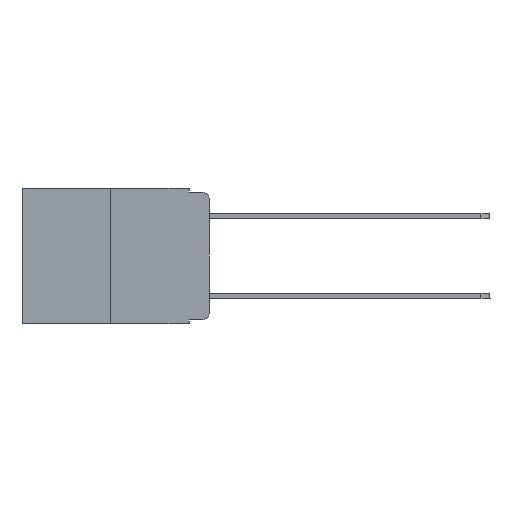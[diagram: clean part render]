
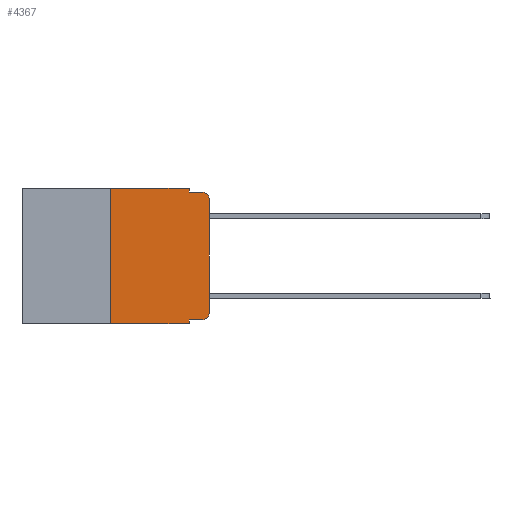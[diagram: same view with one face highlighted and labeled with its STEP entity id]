
A CAD part, left-side view. The second image highlights one B-rep face of the part: STEP entity #4367.
In plain terms, the highlighted planar face has unit normal (-1, 0, 0).
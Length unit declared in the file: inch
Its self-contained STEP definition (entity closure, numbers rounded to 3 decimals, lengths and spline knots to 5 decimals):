
#62 = DIRECTION ( 'NONE',  ( -1., 0., 0. ) ) ;
#111 = CARTESIAN_POINT ( 'NONE',  ( 0., 0.051, -0.01 ) ) ;
#130 = CARTESIAN_POINT ( 'NONE',  ( 0., 0.473, -0.343 ) ) ;
#155 = DIRECTION ( 'NONE',  ( 0., -1., 0. ) ) ;
#194 = EDGE_LOOP ( 'NONE', ( #666, #7816, #8750, #13253, #8079, #11568, #5250, #11345, #1914, #5513 ) ) ;
#237 = CARTESIAN_POINT ( 'NONE',  ( 0., 0.25, -0.343 ) ) ;
#478 = EDGE_CURVE ( 'NONE', #10730, #10467, #6458, .T. ) ;
#509 = VERTEX_POINT ( 'NONE', #9532 ) ;
#565 = CARTESIAN_POINT ( 'NONE',  ( 0., 0.051, -0.01 ) ) ;
#666 = ORIENTED_EDGE ( 'NONE', *, *, #4451, .T. ) ;
#850 = DIRECTION ( 'NONE',  ( 0., 0., -1. ) ) ;
#1027 = CARTESIAN_POINT ( 'NONE',  ( 0., 0.473, 0. ) ) ;
#1044 = VERTEX_POINT ( 'NONE', #565 ) ;
#1249 = CARTESIAN_POINT ( 'NONE',  ( 0., 0.473, 0. ) ) ;
#1609 = CIRCLE ( 'NONE', #9938, 0.02 ) ;
#1702 = CARTESIAN_POINT ( 'NONE',  ( 0., 0., -0.03 ) ) ;
#1792 = VERTEX_POINT ( 'NONE', #237 ) ;
#1804 = EDGE_CURVE ( 'NONE', #10467, #1044, #11845, .T. ) ;
#1914 = ORIENTED_EDGE ( 'NONE', *, *, #2360, .T. ) ;
#2055 = DIRECTION ( 'NONE',  ( 0., 0., -1. ) ) ;
#2360 = EDGE_CURVE ( 'NONE', #12240, #9501, #11832, .T. ) ;
#2678 = LINE ( 'NONE', #111, #7597 ) ;
#2877 = CARTESIAN_POINT ( 'NONE',  ( 0., 0.051, 0. ) ) ;
#2961 = DIRECTION ( 'NONE',  ( 0., -1., 0. ) ) ;
#3334 = LINE ( 'NONE', #13364, #9729 ) ;
#3746 = CARTESIAN_POINT ( 'NONE',  ( 0., 0.02, -0.03 ) ) ;
#4112 = VECTOR ( 'NONE', #2961, 39.37008 ) ;
#4146 = CARTESIAN_POINT ( 'NONE',  ( 0., 0.02, -0.333 ) ) ;
#4367 = ADVANCED_FACE ( 'NONE', ( #7388 ), #13585, .F. ) ;
#4451 = EDGE_CURVE ( 'NONE', #13187, #8229, #13448, .T. ) ;
#4494 = LINE ( 'NONE', #2877, #9239 ) ;
#4852 = CIRCLE ( 'NONE', #10900, 0.02 ) ;
#5008 = VECTOR ( 'NONE', #7662, 39.37008 ) ;
#5040 = CARTESIAN_POINT ( 'NONE',  ( 0., 0.02, -0.01 ) ) ;
#5110 = CARTESIAN_POINT ( 'NONE',  ( 0., 0.051, -0.333 ) ) ;
#5250 = ORIENTED_EDGE ( 'NONE', *, *, #11779, .T. ) ;
#5436 = VECTOR ( 'NONE', #11650, 39.37008 ) ;
#5513 = ORIENTED_EDGE ( 'NONE', *, *, #10539, .T. ) ;
#5868 = DIRECTION ( 'NONE',  ( 0., 0., -1. ) ) ;
#6458 = LINE ( 'NONE', #1249, #12726 ) ;
#7017 = EDGE_CURVE ( 'NONE', #8229, #10085, #4852, .T. ) ;
#7388 = FACE_OUTER_BOUND ( 'NONE', #194, .T. ) ;
#7597 = VECTOR ( 'NONE', #11438, 39.37008 ) ;
#7662 = DIRECTION ( 'NONE',  ( 0., -1., 0. ) ) ;
#7702 = EDGE_CURVE ( 'NONE', #1792, #10730, #3334, .T. ) ;
#7721 = EDGE_CURVE ( 'NONE', #12240, #509, #4494, .T. ) ;
#7727 = EDGE_CURVE ( 'NONE', #1044, #10085, #2678, .T. ) ;
#7816 = ORIENTED_EDGE ( 'NONE', *, *, #7017, .T. ) ;
#8079 = ORIENTED_EDGE ( 'NONE', *, *, #478, .F. ) ;
#8166 = CARTESIAN_POINT ( 'NONE',  ( 0., 0.02, -0.313 ) ) ;
#8229 = VERTEX_POINT ( 'NONE', #1702 ) ;
#8335 = DIRECTION ( 'NONE',  ( 1., 0., 0. ) ) ;
#8611 = CARTESIAN_POINT ( 'NONE',  ( 0., 0., -0.313 ) ) ;
#8750 = ORIENTED_EDGE ( 'NONE', *, *, #7727, .F. ) ;
#9239 = VECTOR ( 'NONE', #850, 39.37008 ) ;
#9501 = VERTEX_POINT ( 'NONE', #4146 ) ;
#9532 = CARTESIAN_POINT ( 'NONE',  ( 0., 0.051, -0.343 ) ) ;
#9571 = DIRECTION ( 'NONE',  ( 0., 0., 1. ) ) ;
#9614 = CARTESIAN_POINT ( 'NONE',  ( 0., 0., 0. ) ) ;
#9729 = VECTOR ( 'NONE', #11251, 39.37008 ) ;
#9938 = AXIS2_PLACEMENT_3D ( 'NONE', #8166, #62, #10141 ) ;
#10085 = VERTEX_POINT ( 'NONE', #5040 ) ;
#10141 = DIRECTION ( 'NONE',  ( 0., 0., -1. ) ) ;
#10433 = CARTESIAN_POINT ( 'NONE',  ( 0., 0.051, -0.333 ) ) ;
#10467 = VERTEX_POINT ( 'NONE', #11281 ) ;
#10539 = EDGE_CURVE ( 'NONE', #9501, #13187, #1609, .T. ) ;
#10596 = CARTESIAN_POINT ( 'NONE',  ( 0., 0.25, 0. ) ) ;
#10730 = VERTEX_POINT ( 'NONE', #10596 ) ;
#10762 = CARTESIAN_POINT ( 'NONE',  ( 0., 0.051, 0. ) ) ;
#10900 = AXIS2_PLACEMENT_3D ( 'NONE', #3746, #12170, #5868 ) ;
#11251 = DIRECTION ( 'NONE',  ( 0., 0., 1. ) ) ;
#11281 = CARTESIAN_POINT ( 'NONE',  ( 0., 0.051, 0. ) ) ;
#11345 = ORIENTED_EDGE ( 'NONE', *, *, #7721, .F. ) ;
#11438 = DIRECTION ( 'NONE',  ( 0., -1., 0. ) ) ;
#11568 = ORIENTED_EDGE ( 'NONE', *, *, #7702, .F. ) ;
#11650 = DIRECTION ( 'NONE',  ( 0., 0., -1. ) ) ;
#11779 = EDGE_CURVE ( 'NONE', #1792, #509, #13381, .T. ) ;
#11832 = LINE ( 'NONE', #10433, #4112 ) ;
#11845 = LINE ( 'NONE', #10762, #5436 ) ;
#12170 = DIRECTION ( 'NONE',  ( -1., 0., 0. ) ) ;
#12199 = AXIS2_PLACEMENT_3D ( 'NONE', #1027, #8335, #2055 ) ;
#12240 = VERTEX_POINT ( 'NONE', #5110 ) ;
#12726 = VECTOR ( 'NONE', #155, 39.37008 ) ;
#12966 = VECTOR ( 'NONE', #9571, 39.37008 ) ;
#13187 = VERTEX_POINT ( 'NONE', #8611 ) ;
#13253 = ORIENTED_EDGE ( 'NONE', *, *, #1804, .F. ) ;
#13364 = CARTESIAN_POINT ( 'NONE',  ( 0., 0.25, 0. ) ) ;
#13381 = LINE ( 'NONE', #130, #5008 ) ;
#13448 = LINE ( 'NONE', #9614, #12966 ) ;
#13585 = PLANE ( 'NONE',  #12199 ) ;
